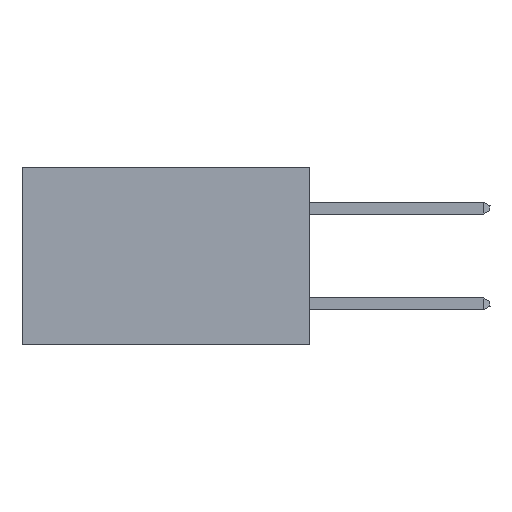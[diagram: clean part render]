
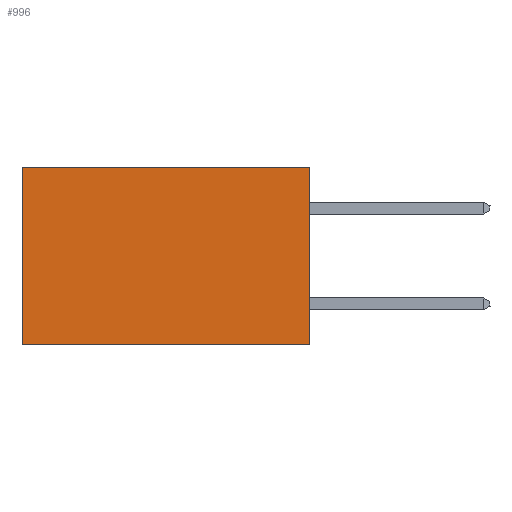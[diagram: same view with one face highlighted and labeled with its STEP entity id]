
A CAD part, left-side view. The second image highlights one B-rep face of the part: STEP entity #996.
In plain terms, the highlighted planar face has unit normal (-1, 0, 0).
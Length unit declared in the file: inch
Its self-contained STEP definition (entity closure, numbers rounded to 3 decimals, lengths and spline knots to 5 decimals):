
#480 = ORIENTED_EDGE ( 'NONE', *, *, #9303, .T. ) ;
#788 = VERTEX_POINT ( 'NONE', #11938 ) ;
#996 = ADVANCED_FACE ( 'NONE', ( #5904 ), #19873, .F. ) ;
#1255 = DIRECTION ( 'NONE',  ( 0., 1., 0. ) ) ;
#1286 = VERTEX_POINT ( 'NONE', #7806 ) ;
#2379 = CARTESIAN_POINT ( 'NONE',  ( 0.2875, 0.6, 0. ) ) ;
#3208 = VERTEX_POINT ( 'NONE', #2379 ) ;
#3904 = DIRECTION ( 'NONE',  ( 0., 1., 0. ) ) ;
#3996 = EDGE_CURVE ( 'NONE', #1286, #15968, #11363, .T. ) ;
#4057 = CARTESIAN_POINT ( 'NONE',  ( 0.2875, 0.6, 0. ) ) ;
#4138 = CARTESIAN_POINT ( 'NONE',  ( 0.2875, 0., -0.37 ) ) ;
#4983 = LINE ( 'NONE', #11998, #15555 ) ;
#5459 = DIRECTION ( 'NONE',  ( 1., 0., 0. ) ) ;
#5691 = CARTESIAN_POINT ( 'NONE',  ( 0.2875, 0., 0. ) ) ;
#5904 = FACE_OUTER_BOUND ( 'NONE', #10305, .T. ) ;
#6934 = EDGE_CURVE ( 'NONE', #15968, #788, #7578, .T. ) ;
#7578 = LINE ( 'NONE', #17768, #14841 ) ;
#7806 = CARTESIAN_POINT ( 'NONE',  ( 0.2875, 0., 0. ) ) ;
#9303 = EDGE_CURVE ( 'NONE', #1286, #3208, #4983, .T. ) ;
#9708 = ORIENTED_EDGE ( 'NONE', *, *, #6934, .F. ) ;
#10305 = EDGE_LOOP ( 'NONE', ( #19337, #9708, #18125, #480 ) ) ;
#11363 = LINE ( 'NONE', #15310, #17771 ) ;
#11938 = CARTESIAN_POINT ( 'NONE',  ( 0.2875, 0.6, -0.37 ) ) ;
#11998 = CARTESIAN_POINT ( 'NONE',  ( 0.2875, 0., 0. ) ) ;
#13307 = LINE ( 'NONE', #4057, #21566 ) ;
#13737 = AXIS2_PLACEMENT_3D ( 'NONE', #5691, #5459, #19738 ) ;
#14841 = VECTOR ( 'NONE', #3904, 39.37008 ) ;
#15310 = CARTESIAN_POINT ( 'NONE',  ( 0.2875, 0., 0. ) ) ;
#15555 = VECTOR ( 'NONE', #1255, 39.37008 ) ;
#15968 = VERTEX_POINT ( 'NONE', #4138 ) ;
#16672 = DIRECTION ( 'NONE',  ( 0., 0., -1. ) ) ;
#17768 = CARTESIAN_POINT ( 'NONE',  ( 0.2875, 0., -0.37 ) ) ;
#17771 = VECTOR ( 'NONE', #20625, 39.37008 ) ;
#18125 = ORIENTED_EDGE ( 'NONE', *, *, #3996, .F. ) ;
#19337 = ORIENTED_EDGE ( 'NONE', *, *, #20312, .T. ) ;
#19738 = DIRECTION ( 'NONE',  ( 0., 0., -1. ) ) ;
#19873 = PLANE ( 'NONE',  #13737 ) ;
#20312 = EDGE_CURVE ( 'NONE', #3208, #788, #13307, .T. ) ;
#20625 = DIRECTION ( 'NONE',  ( 0., 0., -1. ) ) ;
#21566 = VECTOR ( 'NONE', #16672, 39.37008 ) ;
